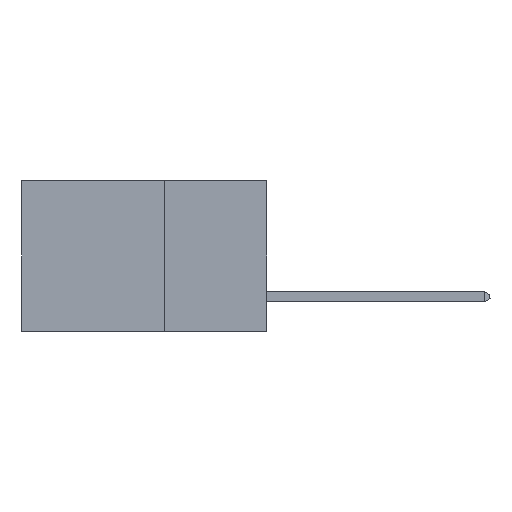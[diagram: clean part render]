
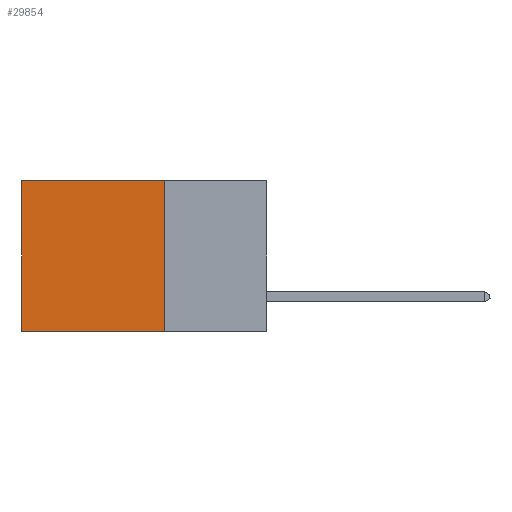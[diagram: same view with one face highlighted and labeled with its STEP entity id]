
A CAD part, left-side view. The second image highlights one B-rep face of the part: STEP entity #29854.
In plain terms, the highlighted planar face has unit normal (-1, 0, 0).
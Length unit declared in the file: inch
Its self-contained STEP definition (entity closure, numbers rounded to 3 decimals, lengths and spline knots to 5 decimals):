
#1772 = DIRECTION ( 'NONE',  ( 0., 0., -1. ) ) ;
#1840 = ORIENTED_EDGE ( 'NONE', *, *, #47553, .T. ) ;
#4586 = VECTOR ( 'NONE', #30945, 39.37008 ) ;
#4798 = LINE ( 'NONE', #5494, #43815 ) ;
#5494 = CARTESIAN_POINT ( 'NONE',  ( 0.2875, 0.25, 0. ) ) ;
#5767 = CARTESIAN_POINT ( 'NONE',  ( 0.2875, 0.25, 0. ) ) ;
#6648 = CARTESIAN_POINT ( 'NONE',  ( 0.2875, 0.25, 0. ) ) ;
#7722 = LINE ( 'NONE', #6648, #48565 ) ;
#11851 = ORIENTED_EDGE ( 'NONE', *, *, #31082, .T. ) ;
#12281 = LINE ( 'NONE', #40096, #37704 ) ;
#16514 = VERTEX_POINT ( 'NONE', #46676 ) ;
#16515 = VERTEX_POINT ( 'NONE', #24157 ) ;
#17577 = VERTEX_POINT ( 'NONE', #44516 ) ;
#19301 = CARTESIAN_POINT ( 'NONE',  ( 0.2875, 0.6, 0. ) ) ;
#22554 = EDGE_CURVE ( 'NONE', #17577, #16514, #12281, .T. ) ;
#24157 = CARTESIAN_POINT ( 'NONE',  ( 0.2875, 0.6, 0. ) ) ;
#25632 = DIRECTION ( 'NONE',  ( 0., 0., -1. ) ) ;
#25850 = LINE ( 'NONE', #19301, #4586 ) ;
#26354 = EDGE_CURVE ( 'NONE', #46779, #17577, #7722, .T. ) ;
#29511 = FACE_OUTER_BOUND ( 'NONE', #48976, .T. ) ;
#29854 = ADVANCED_FACE ( 'NONE', ( #29511 ), #35792, .F. ) ;
#30788 = ORIENTED_EDGE ( 'NONE', *, *, #22554, .F. ) ;
#30945 = DIRECTION ( 'NONE',  ( 0., 0., -1. ) ) ;
#31082 = EDGE_CURVE ( 'NONE', #16515, #16514, #25850, .T. ) ;
#35792 = PLANE ( 'NONE',  #36291 ) ;
#36291 = AXIS2_PLACEMENT_3D ( 'NONE', #5767, #43608, #1772 ) ;
#36590 = CARTESIAN_POINT ( 'NONE',  ( 0.2875, 0.25, 0. ) ) ;
#37704 = VECTOR ( 'NONE', #44081, 39.37008 ) ;
#40096 = CARTESIAN_POINT ( 'NONE',  ( 0.2875, 0.25, -0.37 ) ) ;
#40115 = ORIENTED_EDGE ( 'NONE', *, *, #26354, .F. ) ;
#43608 = DIRECTION ( 'NONE',  ( 1., 0., 0. ) ) ;
#43815 = VECTOR ( 'NONE', #46834, 39.37008 ) ;
#44081 = DIRECTION ( 'NONE',  ( 0., 1., 0. ) ) ;
#44516 = CARTESIAN_POINT ( 'NONE',  ( 0.2875, 0.25, -0.37 ) ) ;
#46676 = CARTESIAN_POINT ( 'NONE',  ( 0.2875, 0.6, -0.37 ) ) ;
#46779 = VERTEX_POINT ( 'NONE', #36590 ) ;
#46834 = DIRECTION ( 'NONE',  ( 0., 1., 0. ) ) ;
#47553 = EDGE_CURVE ( 'NONE', #46779, #16515, #4798, .T. ) ;
#48565 = VECTOR ( 'NONE', #25632, 39.37008 ) ;
#48976 = EDGE_LOOP ( 'NONE', ( #11851, #30788, #40115, #1840 ) ) ;
